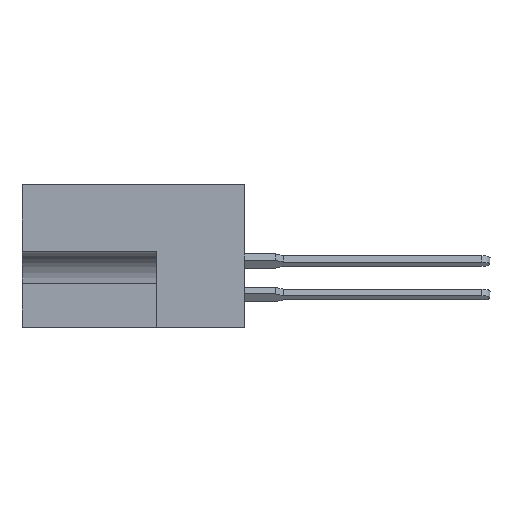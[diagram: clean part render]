
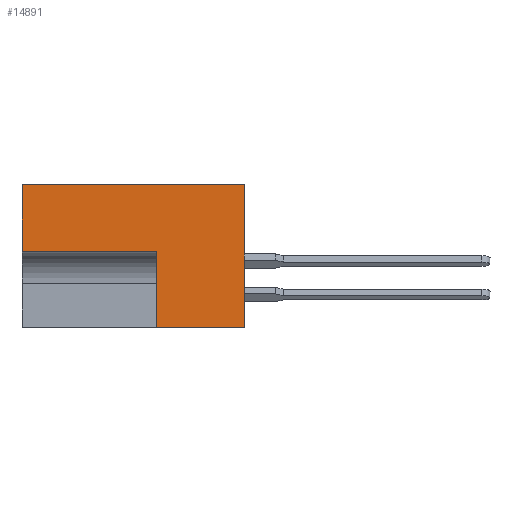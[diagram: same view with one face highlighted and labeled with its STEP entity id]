
A CAD part, left-side view. The second image highlights one B-rep face of the part: STEP entity #14891.
In plain terms, the highlighted planar face has unit normal (-1, 0, 0).
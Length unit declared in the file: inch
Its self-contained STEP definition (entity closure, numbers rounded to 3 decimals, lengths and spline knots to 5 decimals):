
#2 = CARTESIAN_POINT ( 'NONE',  ( 0., 0.328, -0.248 ) ) ;
#509 = CARTESIAN_POINT ( 'NONE',  ( 0., 0.828, 0. ) ) ;
#662 = EDGE_CURVE ( 'NONE', #14880, #14387, #13350, .T. ) ;
#752 = DIRECTION ( 'NONE',  ( 0., 0., -1. ) ) ;
#1049 = EDGE_CURVE ( 'NONE', #14387, #3218, #13138, .T. ) ;
#1206 = DIRECTION ( 'NONE',  ( 0., 0., 1. ) ) ;
#1821 = CARTESIAN_POINT ( 'NONE',  ( 0., 0.453, -0.531 ) ) ;
#1861 = DIRECTION ( 'NONE',  ( 1., 0., 0. ) ) ;
#2034 = CARTESIAN_POINT ( 'NONE',  ( 0., 0.453, 0. ) ) ;
#2128 = EDGE_CURVE ( 'NONE', #10975, #6174, #9283, .T. ) ;
#2711 = LINE ( 'NONE', #10287, #9508 ) ;
#2998 = ORIENTED_EDGE ( 'NONE', *, *, #14552, .F. ) ;
#3136 = VECTOR ( 'NONE', #6187, 39.37008 ) ;
#3218 = VERTEX_POINT ( 'NONE', #3723 ) ;
#3265 = AXIS2_PLACEMENT_3D ( 'NONE', #6859, #1861, #752 ) ;
#3723 = CARTESIAN_POINT ( 'NONE',  ( 0., 0., 0. ) ) ;
#3747 = VECTOR ( 'NONE', #7210, 39.37008 ) ;
#5027 = VECTOR ( 'NONE', #1206, 39.37008 ) ;
#5506 = LINE ( 'NONE', #2034, #3747 ) ;
#5873 = LINE ( 'NONE', #2, #3136 ) ;
#6174 = VERTEX_POINT ( 'NONE', #509 ) ;
#6187 = DIRECTION ( 'NONE',  ( 0., 1., 0. ) ) ;
#6399 = EDGE_LOOP ( 'NONE', ( #15167, #14450, #8736, #13310, #15011, #2998 ) ) ;
#6643 = DIRECTION ( 'NONE',  ( 0., 0., 1. ) ) ;
#6859 = CARTESIAN_POINT ( 'NONE',  ( 0., 0.453, 0. ) ) ;
#6917 = PLANE ( 'NONE',  #3265 ) ;
#7210 = DIRECTION ( 'NONE',  ( 0., -1., 0. ) ) ;
#8125 = VECTOR ( 'NONE', #6643, 39.37008 ) ;
#8666 = CARTESIAN_POINT ( 'NONE',  ( 0., 0., 0. ) ) ;
#8736 = ORIENTED_EDGE ( 'NONE', *, *, #16081, .F. ) ;
#9283 = LINE ( 'NONE', #12886, #8125 ) ;
#9464 = CARTESIAN_POINT ( 'NONE',  ( 0., 0.328, -0.248 ) ) ;
#9508 = VECTOR ( 'NONE', #12870, 39.37008 ) ;
#10127 = FACE_OUTER_BOUND ( 'NONE', #6399, .T. ) ;
#10287 = CARTESIAN_POINT ( 'NONE',  ( 0., 0.328, -0.531 ) ) ;
#10520 = EDGE_CURVE ( 'NONE', #11805, #10975, #5873, .T. ) ;
#10975 = VERTEX_POINT ( 'NONE', #13589 ) ;
#11805 = VERTEX_POINT ( 'NONE', #9464 ) ;
#12870 = DIRECTION ( 'NONE',  ( 0., 0., 1. ) ) ;
#12886 = CARTESIAN_POINT ( 'NONE',  ( 0., 0.828, 0. ) ) ;
#13017 = CARTESIAN_POINT ( 'NONE',  ( 0., 0., -0.531 ) ) ;
#13138 = LINE ( 'NONE', #8666, #5027 ) ;
#13152 = VECTOR ( 'NONE', #14253, 39.37008 ) ;
#13310 = ORIENTED_EDGE ( 'NONE', *, *, #662, .T. ) ;
#13350 = LINE ( 'NONE', #1821, #13152 ) ;
#13589 = CARTESIAN_POINT ( 'NONE',  ( 0., 0.828, -0.248 ) ) ;
#14253 = DIRECTION ( 'NONE',  ( 0., -1., 0. ) ) ;
#14387 = VERTEX_POINT ( 'NONE', #13017 ) ;
#14450 = ORIENTED_EDGE ( 'NONE', *, *, #10520, .F. ) ;
#14552 = EDGE_CURVE ( 'NONE', #6174, #3218, #5506, .T. ) ;
#14880 = VERTEX_POINT ( 'NONE', #15634 ) ;
#14891 = ADVANCED_FACE ( 'NONE', ( #10127 ), #6917, .F. ) ;
#15011 = ORIENTED_EDGE ( 'NONE', *, *, #1049, .T. ) ;
#15167 = ORIENTED_EDGE ( 'NONE', *, *, #2128, .F. ) ;
#15634 = CARTESIAN_POINT ( 'NONE',  ( 0., 0.328, -0.531 ) ) ;
#16081 = EDGE_CURVE ( 'NONE', #14880, #11805, #2711, .T. ) ;
